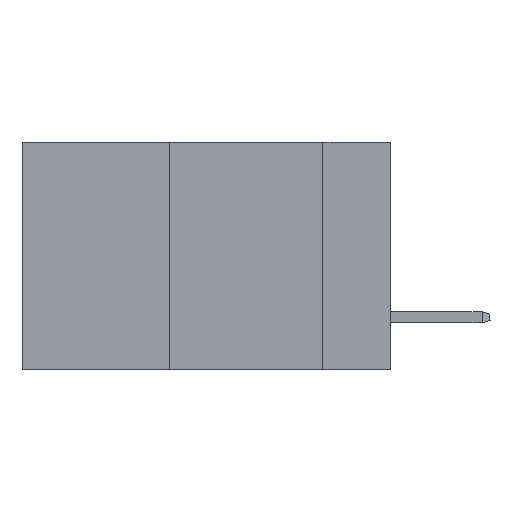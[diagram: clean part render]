
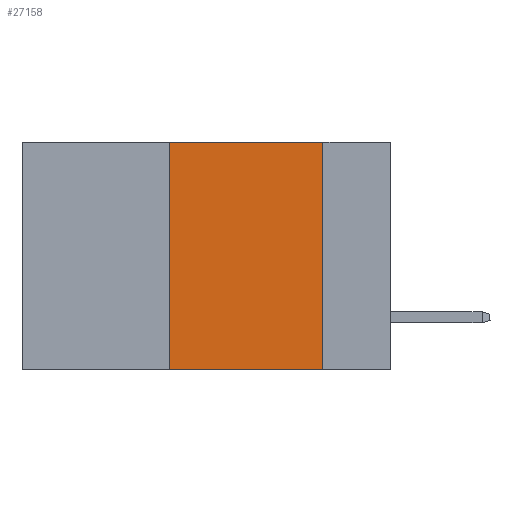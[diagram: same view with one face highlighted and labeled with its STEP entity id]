
A CAD part, left-side view. The second image highlights one B-rep face of the part: STEP entity #27158.
In plain terms, the highlighted planar face has unit normal (-1, 0, 0).
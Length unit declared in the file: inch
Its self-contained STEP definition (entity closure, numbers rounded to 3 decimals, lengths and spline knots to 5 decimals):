
#627 = CARTESIAN_POINT ( 'NONE',  ( 0., 0.11, 0. ) ) ;
#1741 = CARTESIAN_POINT ( 'NONE',  ( 0., 0.6, 0. ) ) ;
#4570 = CARTESIAN_POINT ( 'NONE',  ( 0., 0.11, 0. ) ) ;
#5733 = AXIS2_PLACEMENT_3D ( 'NONE', #1741, #27277, #30122 ) ;
#6489 = CARTESIAN_POINT ( 'NONE',  ( 0., 0.36, -0.37 ) ) ;
#7165 = ORIENTED_EDGE ( 'NONE', *, *, #22864, .F. ) ;
#7341 = FACE_OUTER_BOUND ( 'NONE', #10654, .T. ) ;
#10654 = EDGE_LOOP ( 'NONE', ( #22797, #7165, #34479, #18533 ) ) ;
#12493 = CARTESIAN_POINT ( 'NONE',  ( 0., 0.6, 0. ) ) ;
#14868 = DIRECTION ( 'NONE',  ( 0., 0., -1. ) ) ;
#14925 = VERTEX_POINT ( 'NONE', #4570 ) ;
#15522 = LINE ( 'NONE', #12493, #27956 ) ;
#18533 = ORIENTED_EDGE ( 'NONE', *, *, #29109, .T. ) ;
#19212 = CARTESIAN_POINT ( 'NONE',  ( 0., 0.36, 0. ) ) ;
#20598 = LINE ( 'NONE', #19212, #30854 ) ;
#20704 = VECTOR ( 'NONE', #35855, 39.37008 ) ;
#20928 = VECTOR ( 'NONE', #14868, 39.37008 ) ;
#21037 = VERTEX_POINT ( 'NONE', #6489 ) ;
#21102 = EDGE_CURVE ( 'NONE', #14925, #25493, #26720, .T. ) ;
#22797 = ORIENTED_EDGE ( 'NONE', *, *, #21102, .F. ) ;
#22864 = EDGE_CURVE ( 'NONE', #36226, #14925, #15522, .T. ) ;
#24457 = CARTESIAN_POINT ( 'NONE',  ( 0., 0.6, -0.37 ) ) ;
#25493 = VERTEX_POINT ( 'NONE', #34159 ) ;
#26720 = LINE ( 'NONE', #627, #20928 ) ;
#27158 = ADVANCED_FACE ( 'NONE', ( #7341 ), #35688, .F. ) ;
#27277 = DIRECTION ( 'NONE',  ( 1., 0., 0. ) ) ;
#27418 = LINE ( 'NONE', #24457, #20704 ) ;
#27956 = VECTOR ( 'NONE', #29865, 39.37008 ) ;
#29109 = EDGE_CURVE ( 'NONE', #21037, #25493, #27418, .T. ) ;
#29286 = CARTESIAN_POINT ( 'NONE',  ( 0., 0.36, 0. ) ) ;
#29865 = DIRECTION ( 'NONE',  ( 0., -1., 0. ) ) ;
#30122 = DIRECTION ( 'NONE',  ( 0., 0., -1. ) ) ;
#30526 = DIRECTION ( 'NONE',  ( 0., 0., 1. ) ) ;
#30854 = VECTOR ( 'NONE', #30526, 39.37008 ) ;
#30952 = EDGE_CURVE ( 'NONE', #21037, #36226, #20598, .T. ) ;
#34159 = CARTESIAN_POINT ( 'NONE',  ( 0., 0.11, -0.37 ) ) ;
#34479 = ORIENTED_EDGE ( 'NONE', *, *, #30952, .F. ) ;
#35688 = PLANE ( 'NONE',  #5733 ) ;
#35855 = DIRECTION ( 'NONE',  ( 0., -1., 0. ) ) ;
#36226 = VERTEX_POINT ( 'NONE', #29286 ) ;
